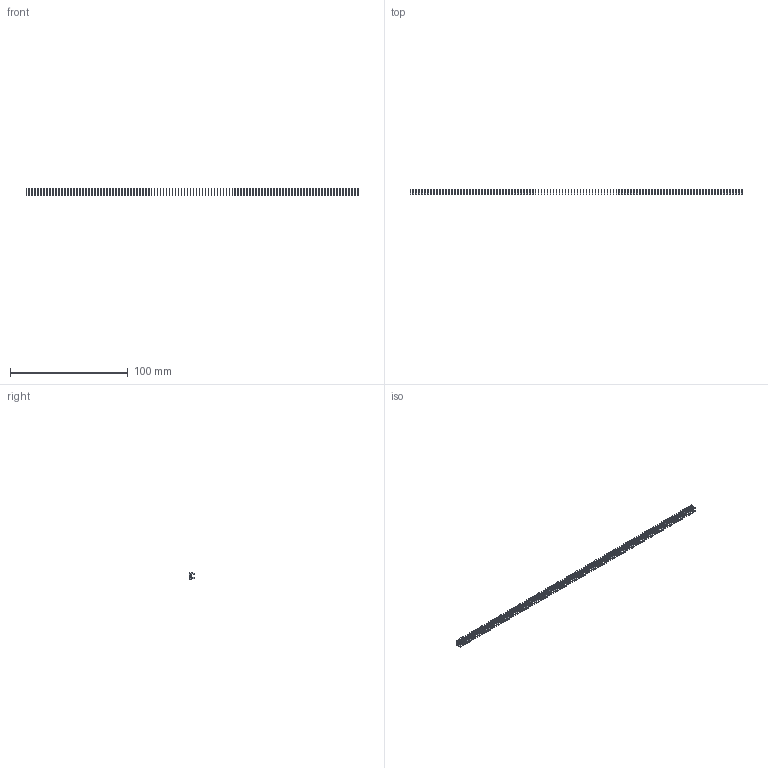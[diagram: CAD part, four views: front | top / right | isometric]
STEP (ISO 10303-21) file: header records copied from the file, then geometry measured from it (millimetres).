
FILE_DESCRIPTION (( 'STEP AP203' ), '1' );
FILE_NAME ('105-112-208-100.STEP', '2020-04-08T01:23:43', ( '' ), ( '' ), 'SwSTEP 2.0', 'SolidWorks 2016', '' );
FILE_SCHEMA (( 'CONFIG_CONTROL_DESIGN' ));
Length unit declared in the file: inch
Products named in the file (2): 100-290-001_100-290-208; 105-112-208-100
Assembly tree (112 placements, depth 2):
  105-112-208-100
    100-290-001_100-290-208  x112
Bounding box: 282.45 x 4.83 x 5.17 mm (x, y, z)
Volume: 770.6 mm3; surface area: 4759.6 mm2
Topology: 112 solids, 112 shells, 2800 faces, 7728 edges, 5152 vertices
Faces by surface type: plane 2464, cylinder 336
Entity records: 4541 total; most frequent: DIRECTION 355, CARTESIAN_POINT 255, COORDINATED_UNIVERSAL_TIME_OFFSET 234, DATE_AND_TIME 234, CALENDAR_DATE 234, LOCAL_TIME 234, AXIS2_PLACEMENT_3D 146, ORIENTED_EDGE 138
